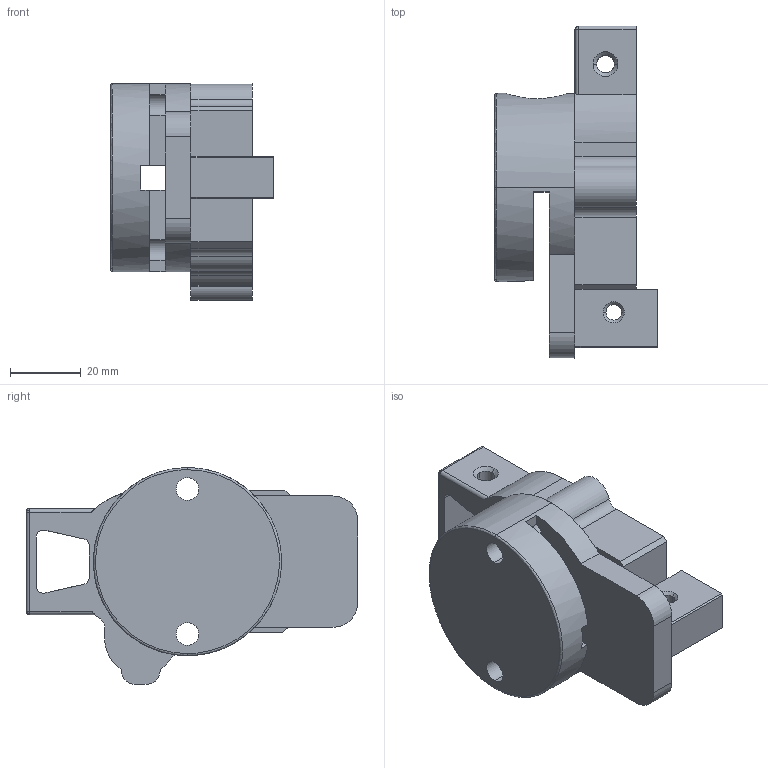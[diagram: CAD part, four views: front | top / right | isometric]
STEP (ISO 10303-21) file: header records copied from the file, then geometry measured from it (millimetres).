
FILE_DESCRIPTION (( 'STEP AP203' ), '1' );
FILE_NAME ('ENDCAP.STEP', '2020-09-28T01:14:10', ( '' ), ( '' ), 'SwSTEP 2.0', 'SolidWorks 2019', '' );
FILE_SCHEMA (( 'CONFIG_CONTROL_DESIGN' ));
Length unit declared in the file: millimetre
Products named in the file (1): ENDCAP
Bounding box: 45.98 x 93.84 x 61.31 mm (x, y, z)
Volume: 92018.5 mm3; surface area: 23544.6 mm2
Topology: 1 solids, 1 shells, 102 faces, 291 edges, 186 vertices
Faces by surface type: plane 48, cylinder 40, cone 8, bspline 6
Entity records: 3616 total; most frequent: CARTESIAN_POINT 816, DIRECTION 581, ORIENTED_EDGE 574, EDGE_CURVE 287, AXIS2_PLACEMENT_3D 207, VERTEX_POINT 186, LINE 167, VECTOR 167
